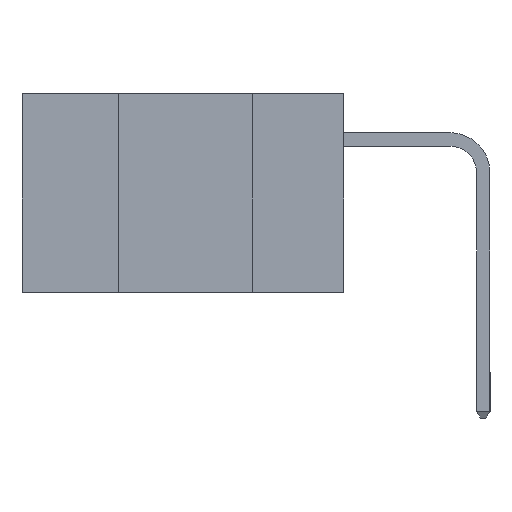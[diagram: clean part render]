
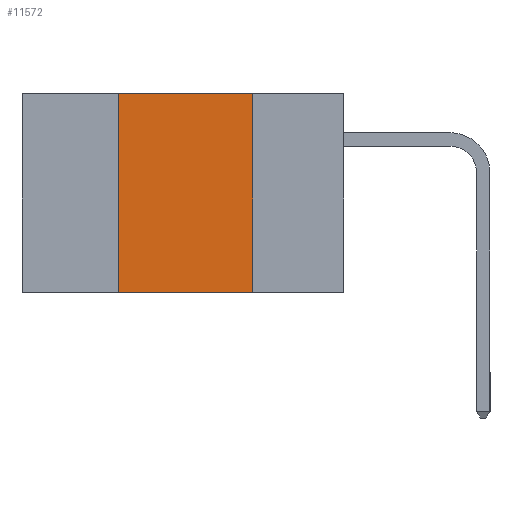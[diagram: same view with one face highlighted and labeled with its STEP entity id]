
A CAD part, left-side view. The second image highlights one B-rep face of the part: STEP entity #11572.
In plain terms, the highlighted planar face has unit normal (-1, 0, 0).
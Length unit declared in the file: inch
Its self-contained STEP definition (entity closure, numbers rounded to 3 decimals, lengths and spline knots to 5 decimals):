
#341 = CARTESIAN_POINT ( 'NONE',  ( 0., 0.6, -0.37 ) ) ;
#493 = DIRECTION ( 'NONE',  ( 0., 0., -1. ) ) ;
#1757 = VERTEX_POINT ( 'NONE', #21058 ) ;
#2690 = LINE ( 'NONE', #6850, #13199 ) ;
#3951 = VERTEX_POINT ( 'NONE', #13368 ) ;
#4232 = AXIS2_PLACEMENT_3D ( 'NONE', #6177, #6278, #8549 ) ;
#4395 = ORIENTED_EDGE ( 'NONE', *, *, #14472, .F. ) ;
#4396 = CARTESIAN_POINT ( 'NONE',  ( 0., 0.42, 0. ) ) ;
#4613 = ORIENTED_EDGE ( 'NONE', *, *, #9906, .F. ) ;
#6177 = CARTESIAN_POINT ( 'NONE',  ( 0., 0.6, 0. ) ) ;
#6278 = DIRECTION ( 'NONE',  ( 1., 0., 0. ) ) ;
#6850 = CARTESIAN_POINT ( 'NONE',  ( 0., 0.17, 0. ) ) ;
#8549 = DIRECTION ( 'NONE',  ( 0., 0., -1. ) ) ;
#9703 = FACE_OUTER_BOUND ( 'NONE', #24447, .T. ) ;
#9906 = EDGE_CURVE ( 'NONE', #27372, #26617, #2690, .T. ) ;
#10823 = EDGE_CURVE ( 'NONE', #3951, #26617, #18692, .T. ) ;
#11572 = ADVANCED_FACE ( 'NONE', ( #9703 ), #28603, .F. ) ;
#12454 = CARTESIAN_POINT ( 'NONE',  ( 0., 0.17, 0. ) ) ;
#13199 = VECTOR ( 'NONE', #493, 39.37008 ) ;
#13288 = DIRECTION ( 'NONE',  ( 0., 0., 1. ) ) ;
#13368 = CARTESIAN_POINT ( 'NONE',  ( 0., 0.42, -0.37 ) ) ;
#13379 = LINE ( 'NONE', #19811, #24882 ) ;
#13592 = DIRECTION ( 'NONE',  ( 0., -1., 0. ) ) ;
#14472 = EDGE_CURVE ( 'NONE', #3951, #1757, #23883, .T. ) ;
#15424 = DIRECTION ( 'NONE',  ( 0., -1., 0. ) ) ;
#17916 = VECTOR ( 'NONE', #13288, 39.37008 ) ;
#18692 = LINE ( 'NONE', #341, #24990 ) ;
#19423 = ORIENTED_EDGE ( 'NONE', *, *, #10823, .T. ) ;
#19811 = CARTESIAN_POINT ( 'NONE',  ( 0., 0.6, 0. ) ) ;
#21058 = CARTESIAN_POINT ( 'NONE',  ( 0., 0.42, 0. ) ) ;
#23883 = LINE ( 'NONE', #4396, #17916 ) ;
#24447 = EDGE_LOOP ( 'NONE', ( #4613, #27766, #4395, #19423 ) ) ;
#24882 = VECTOR ( 'NONE', #15424, 39.37008 ) ;
#24966 = CARTESIAN_POINT ( 'NONE',  ( 0., 0.17, -0.37 ) ) ;
#24990 = VECTOR ( 'NONE', #13592, 39.37008 ) ;
#25183 = EDGE_CURVE ( 'NONE', #1757, #27372, #13379, .T. ) ;
#26617 = VERTEX_POINT ( 'NONE', #24966 ) ;
#27372 = VERTEX_POINT ( 'NONE', #12454 ) ;
#27766 = ORIENTED_EDGE ( 'NONE', *, *, #25183, .F. ) ;
#28603 = PLANE ( 'NONE',  #4232 ) ;
